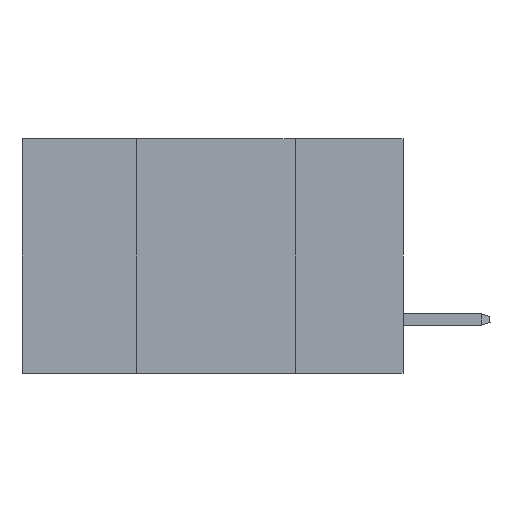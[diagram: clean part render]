
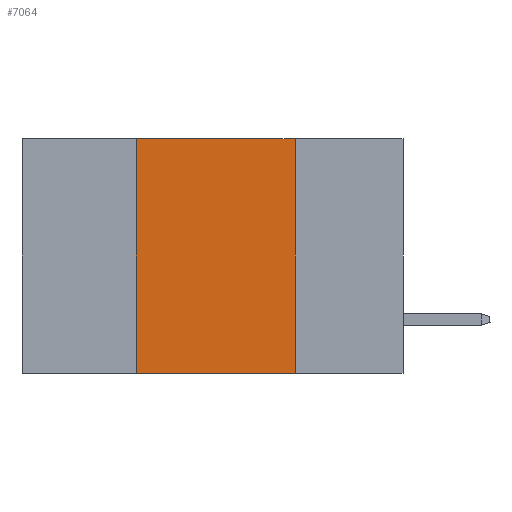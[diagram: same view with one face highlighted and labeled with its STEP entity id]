
A CAD part, left-side view. The second image highlights one B-rep face of the part: STEP entity #7064.
In plain terms, the highlighted planar face has unit normal (-1, 0, 0).
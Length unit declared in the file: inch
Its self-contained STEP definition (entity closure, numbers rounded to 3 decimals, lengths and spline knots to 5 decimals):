
#1000 = LINE ( 'NONE', #22455, #1850 ) ;
#1034 = CARTESIAN_POINT ( 'NONE',  ( 0., 0.42, 0. ) ) ;
#1850 = VECTOR ( 'NONE', #22578, 39.37008 ) ;
#1910 = DIRECTION ( 'NONE',  ( 0., 0., -1. ) ) ;
#2429 = CARTESIAN_POINT ( 'NONE',  ( 0., 0.42, -0.37 ) ) ;
#2431 = AXIS2_PLACEMENT_3D ( 'NONE', #21598, #14255, #5445 ) ;
#3102 = LINE ( 'NONE', #10342, #5462 ) ;
#3496 = ORIENTED_EDGE ( 'NONE', *, *, #20451, .F. ) ;
#5445 = DIRECTION ( 'NONE',  ( 0., 0., -1. ) ) ;
#5462 = VECTOR ( 'NONE', #19128, 39.37008 ) ;
#5539 = CARTESIAN_POINT ( 'NONE',  ( 0., 0.17, 0. ) ) ;
#5852 = EDGE_LOOP ( 'NONE', ( #3496, #11794, #14608, #19553 ) ) ;
#5995 = EDGE_CURVE ( 'NONE', #9147, #10114, #3102, .T. ) ;
#6294 = CARTESIAN_POINT ( 'NONE',  ( 0., 0.6, 0. ) ) ;
#6723 = VECTOR ( 'NONE', #1910, 39.37008 ) ;
#7064 = ADVANCED_FACE ( 'NONE', ( #17755 ), #7299, .F. ) ;
#7299 = PLANE ( 'NONE',  #2431 ) ;
#9147 = VERTEX_POINT ( 'NONE', #2429 ) ;
#9847 = CARTESIAN_POINT ( 'NONE',  ( 0., 0.17, -0.37 ) ) ;
#10114 = VERTEX_POINT ( 'NONE', #9847 ) ;
#10342 = CARTESIAN_POINT ( 'NONE',  ( 0., 0.6, -0.37 ) ) ;
#10817 = LINE ( 'NONE', #5539, #6723 ) ;
#11794 = ORIENTED_EDGE ( 'NONE', *, *, #22377, .F. ) ;
#13412 = CARTESIAN_POINT ( 'NONE',  ( 0., 0.17, 0. ) ) ;
#13586 = DIRECTION ( 'NONE',  ( 0., -1., 0. ) ) ;
#14255 = DIRECTION ( 'NONE',  ( 1., 0., 0. ) ) ;
#14608 = ORIENTED_EDGE ( 'NONE', *, *, #18611, .F. ) ;
#15432 = VECTOR ( 'NONE', #13586, 39.37008 ) ;
#17181 = VERTEX_POINT ( 'NONE', #13412 ) ;
#17755 = FACE_OUTER_BOUND ( 'NONE', #5852, .T. ) ;
#18611 = EDGE_CURVE ( 'NONE', #9147, #19844, #1000, .T. ) ;
#19128 = DIRECTION ( 'NONE',  ( 0., -1., 0. ) ) ;
#19553 = ORIENTED_EDGE ( 'NONE', *, *, #5995, .T. ) ;
#19844 = VERTEX_POINT ( 'NONE', #1034 ) ;
#20451 = EDGE_CURVE ( 'NONE', #17181, #10114, #10817, .T. ) ;
#21598 = CARTESIAN_POINT ( 'NONE',  ( 0., 0.6, 0. ) ) ;
#22377 = EDGE_CURVE ( 'NONE', #19844, #17181, #22473, .T. ) ;
#22455 = CARTESIAN_POINT ( 'NONE',  ( 0., 0.42, 0. ) ) ;
#22473 = LINE ( 'NONE', #6294, #15432 ) ;
#22578 = DIRECTION ( 'NONE',  ( 0., 0., 1. ) ) ;
